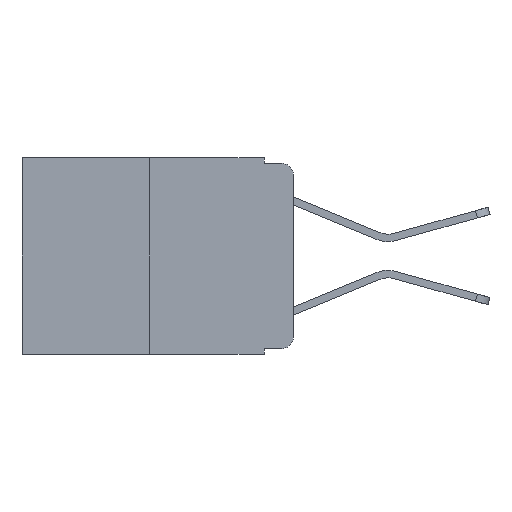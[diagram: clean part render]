
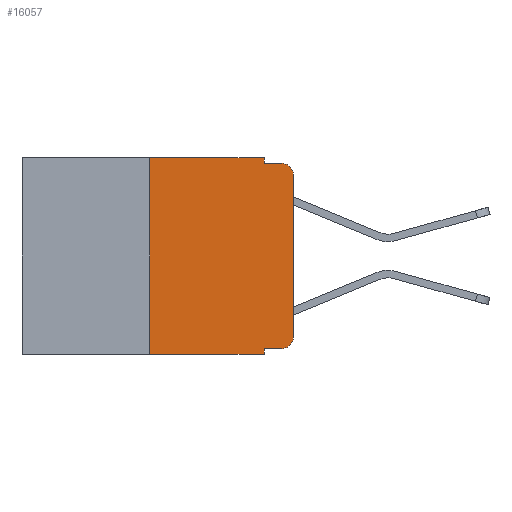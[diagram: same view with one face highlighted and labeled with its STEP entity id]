
A CAD part, left-side view. The second image highlights one B-rep face of the part: STEP entity #16057.
In plain terms, the highlighted planar face has unit normal (-1, 0, 0).
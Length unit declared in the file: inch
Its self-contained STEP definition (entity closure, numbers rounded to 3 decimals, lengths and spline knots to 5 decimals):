
#294 = VERTEX_POINT ( 'NONE', #1769 ) ;
#1510 = AXIS2_PLACEMENT_3D ( 'NONE', #7285, #7211, #10253 ) ;
#1563 = AXIS2_PLACEMENT_3D ( 'NONE', #11750, #7179, #7447 ) ;
#1702 = ORIENTED_EDGE ( 'NONE', *, *, #8002, .F. ) ;
#1769 = CARTESIAN_POINT ( 'NONE',  ( 0., 0., -0.313 ) ) ;
#2021 = VERTEX_POINT ( 'NONE', #14618 ) ;
#2094 = LINE ( 'NONE', #13628, #11472 ) ;
#2449 = DIRECTION ( 'NONE',  ( 0., -1., 0. ) ) ;
#2520 = CARTESIAN_POINT ( 'NONE',  ( 0., 0.25, -0.343 ) ) ;
#2568 = ORIENTED_EDGE ( 'NONE', *, *, #8054, .T. ) ;
#2682 = CARTESIAN_POINT ( 'NONE',  ( 0., 0.051, -0.333 ) ) ;
#2708 = VERTEX_POINT ( 'NONE', #14119 ) ;
#2719 = VECTOR ( 'NONE', #2449, 39.37008 ) ;
#3046 = VERTEX_POINT ( 'NONE', #9035 ) ;
#3127 = VERTEX_POINT ( 'NONE', #2520 ) ;
#3175 = CARTESIAN_POINT ( 'NONE',  ( 0., 0.473, -0.343 ) ) ;
#3360 = VECTOR ( 'NONE', #5151, 39.37008 ) ;
#3481 = CARTESIAN_POINT ( 'NONE',  ( 0., 0.051, -0.01 ) ) ;
#3766 = LINE ( 'NONE', #5478, #10092 ) ;
#4174 = LINE ( 'NONE', #5023, #7133 ) ;
#4283 = CARTESIAN_POINT ( 'NONE',  ( 0., 0.051, 0. ) ) ;
#4929 = CARTESIAN_POINT ( 'NONE',  ( 0., 0.051, -0.343 ) ) ;
#4979 = AXIS2_PLACEMENT_3D ( 'NONE', #9171, #11650, #11707 ) ;
#5023 = CARTESIAN_POINT ( 'NONE',  ( 0., 0.051, 0. ) ) ;
#5151 = DIRECTION ( 'NONE',  ( 0., 0., -1. ) ) ;
#5172 = CIRCLE ( 'NONE', #1563, 0.02 ) ;
#5213 = DIRECTION ( 'NONE',  ( 0., 0., 1. ) ) ;
#5478 = CARTESIAN_POINT ( 'NONE',  ( 0., 0.25, 0. ) ) ;
#6228 = ORIENTED_EDGE ( 'NONE', *, *, #7297, .F. ) ;
#6464 = VERTEX_POINT ( 'NONE', #4929 ) ;
#6497 = VERTEX_POINT ( 'NONE', #3481 ) ;
#7133 = VECTOR ( 'NONE', #11068, 39.37008 ) ;
#7179 = DIRECTION ( 'NONE',  ( -1., 0., 0. ) ) ;
#7211 = DIRECTION ( 'NONE',  ( -1., 0., 0. ) ) ;
#7285 = CARTESIAN_POINT ( 'NONE',  ( 0., 0.02, -0.313 ) ) ;
#7297 = EDGE_CURVE ( 'NONE', #13098, #8787, #8718, .T. ) ;
#7447 = DIRECTION ( 'NONE',  ( 0., 0., -1. ) ) ;
#7505 = LINE ( 'NONE', #10645, #13775 ) ;
#7569 = EDGE_CURVE ( 'NONE', #3127, #6464, #16006, .T. ) ;
#7984 = EDGE_CURVE ( 'NONE', #294, #2021, #2094, .T. ) ;
#7988 = EDGE_CURVE ( 'NONE', #2021, #14587, #5172, .T. ) ;
#8002 = EDGE_CURVE ( 'NONE', #6497, #14587, #7505, .T. ) ;
#8010 = EDGE_CURVE ( 'NONE', #8787, #6497, #4174, .T. ) ;
#8014 = CARTESIAN_POINT ( 'NONE',  ( 0., 0.051, 0. ) ) ;
#8029 = EDGE_CURVE ( 'NONE', #3127, #13098, #3766, .T. ) ;
#8032 = EDGE_CURVE ( 'NONE', #2708, #6464, #13393, .T. ) ;
#8052 = EDGE_CURVE ( 'NONE', #2708, #3046, #10883, .T. ) ;
#8054 = EDGE_CURVE ( 'NONE', #3046, #294, #16163, .T. ) ;
#8316 = VECTOR ( 'NONE', #9459, 39.37008 ) ;
#8556 = ORIENTED_EDGE ( 'NONE', *, *, #8029, .F. ) ;
#8559 = EDGE_LOOP ( 'NONE', ( #16159, #15086, #1702, #15286, #6228, #8556, #12605, #11623, #10437, #2568 ) ) ;
#8718 = LINE ( 'NONE', #12302, #8316 ) ;
#8787 = VERTEX_POINT ( 'NONE', #4283 ) ;
#9035 = CARTESIAN_POINT ( 'NONE',  ( 0., 0.02, -0.333 ) ) ;
#9171 = CARTESIAN_POINT ( 'NONE',  ( 0., 0.473, 0. ) ) ;
#9459 = DIRECTION ( 'NONE',  ( 0., -1., 0. ) ) ;
#10092 = VECTOR ( 'NONE', #5213, 39.37008 ) ;
#10253 = DIRECTION ( 'NONE',  ( 0., 0., -1. ) ) ;
#10373 = DIRECTION ( 'NONE',  ( 0., -1., 0. ) ) ;
#10437 = ORIENTED_EDGE ( 'NONE', *, *, #8052, .T. ) ;
#10452 = PLANE ( 'NONE',  #4979 ) ;
#10645 = CARTESIAN_POINT ( 'NONE',  ( 0., 0.051, -0.01 ) ) ;
#10699 = FACE_OUTER_BOUND ( 'NONE', #8559, .T. ) ;
#10883 = LINE ( 'NONE', #2682, #13009 ) ;
#11068 = DIRECTION ( 'NONE',  ( 0., 0., -1. ) ) ;
#11472 = VECTOR ( 'NONE', #13196, 39.37008 ) ;
#11623 = ORIENTED_EDGE ( 'NONE', *, *, #8032, .F. ) ;
#11650 = DIRECTION ( 'NONE',  ( 1., 0., 0. ) ) ;
#11707 = DIRECTION ( 'NONE',  ( 0., 0., -1. ) ) ;
#11750 = CARTESIAN_POINT ( 'NONE',  ( 0., 0.02, -0.03 ) ) ;
#12302 = CARTESIAN_POINT ( 'NONE',  ( 0., 0.473, 0. ) ) ;
#12568 = CARTESIAN_POINT ( 'NONE',  ( 0., 0.02, -0.01 ) ) ;
#12605 = ORIENTED_EDGE ( 'NONE', *, *, #7569, .T. ) ;
#12858 = CARTESIAN_POINT ( 'NONE',  ( 0., 0.25, 0. ) ) ;
#13009 = VECTOR ( 'NONE', #10373, 39.37008 ) ;
#13098 = VERTEX_POINT ( 'NONE', #12858 ) ;
#13192 = DIRECTION ( 'NONE',  ( 0., -1., 0. ) ) ;
#13196 = DIRECTION ( 'NONE',  ( 0., 0., 1. ) ) ;
#13393 = LINE ( 'NONE', #8014, #3360 ) ;
#13628 = CARTESIAN_POINT ( 'NONE',  ( 0., 0., 0. ) ) ;
#13775 = VECTOR ( 'NONE', #13192, 39.37008 ) ;
#14119 = CARTESIAN_POINT ( 'NONE',  ( 0., 0.051, -0.333 ) ) ;
#14587 = VERTEX_POINT ( 'NONE', #12568 ) ;
#14618 = CARTESIAN_POINT ( 'NONE',  ( 0., 0., -0.03 ) ) ;
#15086 = ORIENTED_EDGE ( 'NONE', *, *, #7988, .T. ) ;
#15286 = ORIENTED_EDGE ( 'NONE', *, *, #8010, .F. ) ;
#16006 = LINE ( 'NONE', #3175, #2719 ) ;
#16057 = ADVANCED_FACE ( 'NONE', ( #10699 ), #10452, .F. ) ;
#16159 = ORIENTED_EDGE ( 'NONE', *, *, #7984, .T. ) ;
#16163 = CIRCLE ( 'NONE', #1510, 0.02 ) ;
